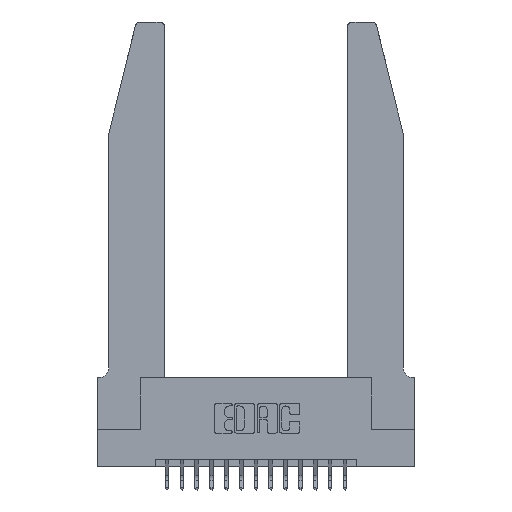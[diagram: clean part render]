
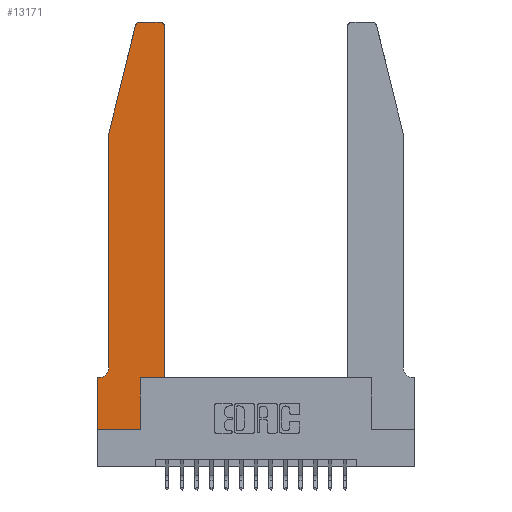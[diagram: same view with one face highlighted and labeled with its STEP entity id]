
A CAD part, top view. The second image highlights one B-rep face of the part: STEP entity #13171.
In plain terms, the highlighted planar face has unit normal (0, 0, 1).
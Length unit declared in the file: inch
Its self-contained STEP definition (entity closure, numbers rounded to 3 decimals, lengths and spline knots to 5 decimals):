
#44 = DIRECTION ( 'NONE',  ( 0., 1., 0. ) ) ;
#116 = EDGE_CURVE ( 'NONE', #14103, #10050, #10699, .T. ) ;
#127 = VERTEX_POINT ( 'NONE', #4462 ) ;
#302 = VERTEX_POINT ( 'NONE', #2572 ) ;
#423 = ORIENTED_EDGE ( 'NONE', *, *, #116, .T. ) ;
#592 = EDGE_CURVE ( 'NONE', #13626, #4260, #3747, .T. ) ;
#807 = CARTESIAN_POINT ( 'NONE',  ( 0.2865, 0.35, 0.37 ) ) ;
#846 = EDGE_CURVE ( 'NONE', #8593, #14322, #11328, .T. ) ;
#1326 = CARTESIAN_POINT ( 'NONE',  ( 0., 0., 0.37 ) ) ;
#1431 = ORIENTED_EDGE ( 'NONE', *, *, #4168, .T. ) ;
#1455 = CARTESIAN_POINT ( 'NONE',  ( 0.2605, 2.75, 0.37 ) ) ;
#2096 = CARTESIAN_POINT ( 'NONE',  ( 0., 0.35, 0.37 ) ) ;
#2493 = CARTESIAN_POINT ( 'NONE',  ( 0.0755, 0.35, 0.37 ) ) ;
#2572 = CARTESIAN_POINT ( 'NONE',  ( 0.0055, 0.35, 0.37 ) ) ;
#3043 = EDGE_CURVE ( 'NONE', #14071, #18140, #7219, .T. ) ;
#3103 = AXIS2_PLACEMENT_3D ( 'NONE', #16963, #10135, #16571 ) ;
#3451 = LINE ( 'NONE', #7644, #10854 ) ;
#3699 = DIRECTION ( 'NONE',  ( 1., 0., 0. ) ) ;
#3700 = VECTOR ( 'NONE', #17012, 39.37008 ) ;
#3747 = CIRCLE ( 'NONE', #3103, 0.03 ) ;
#4168 = EDGE_CURVE ( 'NONE', #18516, #18817, #6474, .T. ) ;
#4177 = DIRECTION ( 'NONE',  ( 0., 0., -1. ) ) ;
#4260 = VERTEX_POINT ( 'NONE', #11679 ) ;
#4304 = VECTOR ( 'NONE', #16110, 39.37008 ) ;
#4462 = CARTESIAN_POINT ( 'NONE',  ( 0.4205, 2.75, 0.37 ) ) ;
#5024 = CARTESIAN_POINT ( 'NONE',  ( 0.0755, 2., 0.37 ) ) ;
#5115 = ORIENTED_EDGE ( 'NONE', *, *, #10446, .T. ) ;
#5429 = CARTESIAN_POINT ( 'NONE',  ( 0.0755, 2., 0.37 ) ) ;
#5584 = ORIENTED_EDGE ( 'NONE', *, *, #18487, .T. ) ;
#6474 = LINE ( 'NONE', #14369, #14160 ) ;
#6816 = VECTOR ( 'NONE', #17252, 39.37008 ) ;
#6877 = CARTESIAN_POINT ( 'NONE',  ( 0., 0., 0.37 ) ) ;
#7219 = LINE ( 'NONE', #10654, #18218 ) ;
#7243 = DIRECTION ( 'NONE',  ( 0., 0., 1. ) ) ;
#7285 = CIRCLE ( 'NONE', #8297, 0.03 ) ;
#7359 = EDGE_CURVE ( 'NONE', #14322, #14071, #15410, .T. ) ;
#7644 = CARTESIAN_POINT ( 'NONE',  ( 0.0755, 2., 0.37 ) ) ;
#7932 = EDGE_CURVE ( 'NONE', #18140, #127, #7285, .T. ) ;
#8297 = AXIS2_PLACEMENT_3D ( 'NONE', #15870, #7243, #17294 ) ;
#8593 = VERTEX_POINT ( 'NONE', #18134 ) ;
#8767 = DIRECTION ( 'NONE',  ( 0., 1., 0. ) ) ;
#9109 = DIRECTION ( 'NONE',  ( -0.239, -0.971, 0. ) ) ;
#9309 = CARTESIAN_POINT ( 'NONE',  ( 0.4505, 0.35, 0.37 ) ) ;
#9480 = CARTESIAN_POINT ( 'NONE',  ( 0.2865, 0.35, 0.37 ) ) ;
#9916 = ORIENTED_EDGE ( 'NONE', *, *, #846, .T. ) ;
#10036 = DIRECTION ( 'NONE',  ( 0., -1., 0. ) ) ;
#10050 = VERTEX_POINT ( 'NONE', #14838 ) ;
#10135 = DIRECTION ( 'NONE',  ( 0., 0., 1. ) ) ;
#10306 = DIRECTION ( 'NONE',  ( 1., 0., 0. ) ) ;
#10446 = EDGE_CURVE ( 'NONE', #302, #18516, #18650, .T. ) ;
#10489 = LINE ( 'NONE', #1455, #18078 ) ;
#10654 = CARTESIAN_POINT ( 'NONE',  ( 0.4505, 0.35, 0.37 ) ) ;
#10698 = EDGE_CURVE ( 'NONE', #4260, #14103, #3451, .T. ) ;
#10699 = LINE ( 'NONE', #5429, #6816 ) ;
#10854 = VECTOR ( 'NONE', #9109, 39.37008 ) ;
#10984 = CARTESIAN_POINT ( 'NONE',  ( 0.284, 2.75, 0.37 ) ) ;
#11328 = LINE ( 'NONE', #9480, #14698 ) ;
#11614 = VECTOR ( 'NONE', #10306, 39.37008 ) ;
#11679 = CARTESIAN_POINT ( 'NONE',  ( 0.25487, 2.72718, 0.37 ) ) ;
#11933 = DIRECTION ( 'NONE',  ( -1., 0., 0. ) ) ;
#12206 = AXIS2_PLACEMENT_3D ( 'NONE', #2096, #12515, #3699 ) ;
#12515 = DIRECTION ( 'NONE',  ( 0., 0., 1. ) ) ;
#12936 = CARTESIAN_POINT ( 'NONE',  ( 0.0055, 0.42, 0.37 ) ) ;
#13171 = ADVANCED_FACE ( 'NONE', ( #13968 ), #18155, .T. ) ;
#13626 = VERTEX_POINT ( 'NONE', #10984 ) ;
#13747 = ORIENTED_EDGE ( 'NONE', *, *, #7359, .T. ) ;
#13968 = FACE_OUTER_BOUND ( 'NONE', #15395, .T. ) ;
#14071 = VERTEX_POINT ( 'NONE', #9309 ) ;
#14103 = VERTEX_POINT ( 'NONE', #5024 ) ;
#14160 = VECTOR ( 'NONE', #10036, 39.37008 ) ;
#14322 = VERTEX_POINT ( 'NONE', #807 ) ;
#14355 = DIRECTION ( 'NONE',  ( -1., 0., 0. ) ) ;
#14369 = CARTESIAN_POINT ( 'NONE',  ( 0., 0., 0.37 ) ) ;
#14628 = ORIENTED_EDGE ( 'NONE', *, *, #7932, .T. ) ;
#14698 = VECTOR ( 'NONE', #8767, 39.37008 ) ;
#14755 = CIRCLE ( 'NONE', #18196, 0.07 ) ;
#14838 = CARTESIAN_POINT ( 'NONE',  ( 0.0755, 0.42, 0.37 ) ) ;
#14843 = ORIENTED_EDGE ( 'NONE', *, *, #18827, .T. ) ;
#15287 = CARTESIAN_POINT ( 'NONE',  ( 0.4505, 2.72, 0.37 ) ) ;
#15292 = ORIENTED_EDGE ( 'NONE', *, *, #592, .T. ) ;
#15395 = EDGE_LOOP ( 'NONE', ( #14843, #15292, #15752, #423, #16211, #5115, #1431, #5584, #9916, #13747, #17974, #14628 ) ) ;
#15410 = LINE ( 'NONE', #17494, #11614 ) ;
#15752 = ORIENTED_EDGE ( 'NONE', *, *, #10698, .T. ) ;
#15870 = CARTESIAN_POINT ( 'NONE',  ( 0.4205, 2.72, 0.37 ) ) ;
#15879 = LINE ( 'NONE', #1326, #4304 ) ;
#16110 = DIRECTION ( 'NONE',  ( 1., 0., 0. ) ) ;
#16211 = ORIENTED_EDGE ( 'NONE', *, *, #18339, .T. ) ;
#16571 = DIRECTION ( 'NONE',  ( 1., 0., 0. ) ) ;
#16963 = CARTESIAN_POINT ( 'NONE',  ( 0.284, 2.72, 0.37 ) ) ;
#17012 = DIRECTION ( 'NONE',  ( -1., 0., 0. ) ) ;
#17252 = DIRECTION ( 'NONE',  ( 0., -1., 0. ) ) ;
#17294 = DIRECTION ( 'NONE',  ( 1., 0., 0. ) ) ;
#17494 = CARTESIAN_POINT ( 'NONE',  ( 0.4505, 0.35, 0.37 ) ) ;
#17523 = CARTESIAN_POINT ( 'NONE',  ( 0., 0.35, 0.37 ) ) ;
#17974 = ORIENTED_EDGE ( 'NONE', *, *, #3043, .T. ) ;
#18078 = VECTOR ( 'NONE', #11933, 39.37008 ) ;
#18134 = CARTESIAN_POINT ( 'NONE',  ( 0.2865, 0., 0.37 ) ) ;
#18140 = VERTEX_POINT ( 'NONE', #15287 ) ;
#18155 = PLANE ( 'NONE',  #12206 ) ;
#18196 = AXIS2_PLACEMENT_3D ( 'NONE', #12936, #4177, #14355 ) ;
#18218 = VECTOR ( 'NONE', #44, 39.37008 ) ;
#18339 = EDGE_CURVE ( 'NONE', #10050, #302, #14755, .T. ) ;
#18487 = EDGE_CURVE ( 'NONE', #18817, #8593, #15879, .T. ) ;
#18516 = VERTEX_POINT ( 'NONE', #17523 ) ;
#18650 = LINE ( 'NONE', #2493, #3700 ) ;
#18817 = VERTEX_POINT ( 'NONE', #6877 ) ;
#18827 = EDGE_CURVE ( 'NONE', #127, #13626, #10489, .T. ) ;
